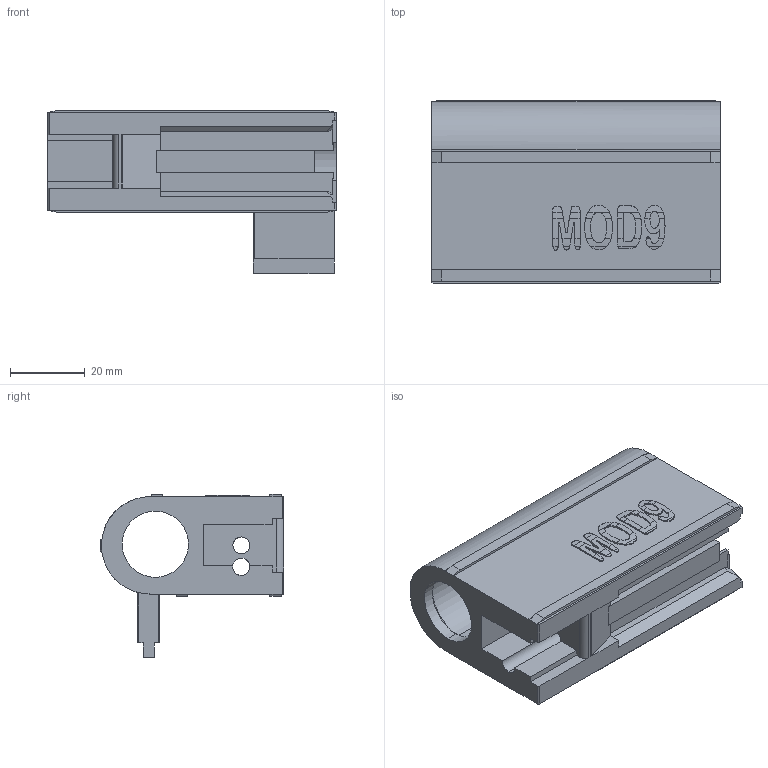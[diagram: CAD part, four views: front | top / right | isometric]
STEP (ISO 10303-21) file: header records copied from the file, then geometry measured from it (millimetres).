
FILE_DESCRIPTION (( 'STEP AP203' ), '1' );
FILE_NAME ('MOD9_V3__Bolt_Carrier.STEP', '2020-12-23T19:27:11', ( '' ), ( '' ), 'SwSTEP 2.0', 'SolidWorks 2019', '' );
FILE_SCHEMA (( 'CONFIG_CONTROL_DESIGN' ));
Length unit declared in the file: millimetre
Products named in the file (1): MOD9_V3__Bolt_Carrier
Bounding box: 77.19 x 48.98 x 43.65 mm (x, y, z)
Volume: 47871.6 mm3; surface area: 22287.2 mm2
Topology: 1 solids, 1 shells, 292 faces, 837 edges, 550 vertices
Faces by surface type: plane 135, bspline 133, cylinder 22, cone 2
Entity records: 11998 total; most frequent: CARTESIAN_POINT 5328, ORIENTED_EDGE 1674, DIRECTION 860, EDGE_CURVE 837, VERTEX_POINT 550, VECTOR 470, LINE 470, B_SPLINE_CURVE_WITH_KNOTS 329
